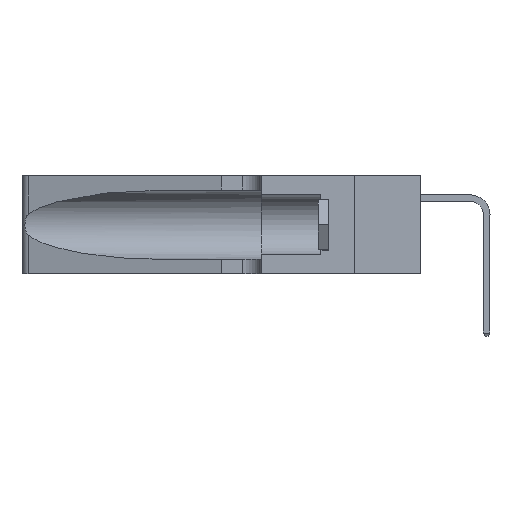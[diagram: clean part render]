
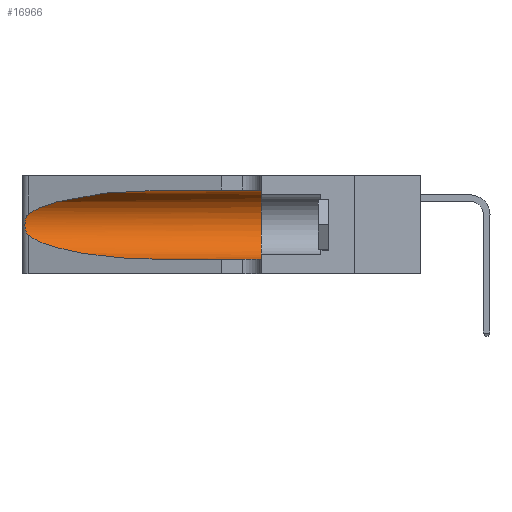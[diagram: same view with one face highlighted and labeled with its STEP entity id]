
A CAD part, left-side view. The second image highlights one B-rep face of the part: STEP entity #16966.
In plain terms, the highlighted cylindrical face has radius 3.308 mm (diameter 6.617 mm), a partial arc.
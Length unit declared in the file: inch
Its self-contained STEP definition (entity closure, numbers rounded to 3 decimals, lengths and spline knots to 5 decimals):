
#611 = FACE_OUTER_BOUND ( 'NONE', #4443, .T. ) ;
#822 = EDGE_CURVE ( 'NONE', #9810, #2990, #13252, .T. ) ;
#973 = CARTESIAN_POINT ( 'NONE',  ( 0.26017, 1.23833, 0.17102 ) ) ;
#1221 = B_SPLINE_CURVE_WITH_KNOTS ( 'NONE', 3,
 ( #13715, #10117, #19068, #8324, #20815, #10199, #22566, #11981, #973, #13793, #2864, #15622, #4724, #17380 ),
 .UNSPECIFIED., .F., .F.,
 ( 4, 2, 2, 2, 2, 2, 4 ),
 ( 0., 0.00027, 0.00053, 0.00107, 0.0016, 0.00187, 0.00214 ),
 .UNSPECIFIED. ) ;
#1453 = CARTESIAN_POINT ( 'NONE',  ( 0.25487, 1.22718, 0.14631 ) ) ;
#1502 = CIRCLE ( 'NONE', #5967, 0.13025 ) ;
#2205 = ORIENTED_EDGE ( 'NONE', *, *, #14631, .T. ) ;
#2864 = CARTESIAN_POINT ( 'NONE',  ( 0.25789, 1.23486, 0.15765 ) ) ;
#2990 = VERTEX_POINT ( 'NONE', #14457 ) ;
#3631 = EDGE_CURVE ( 'NONE', #18304, #9810, #9086, .T. ) ;
#3703 = DIRECTION ( 'NONE',  ( 0., -1., 0. ) ) ;
#4443 = EDGE_LOOP ( 'NONE', ( #17193, #2205, #8664, #22446, #21426, #20558 ) ) ;
#4724 = CARTESIAN_POINT ( 'NONE',  ( 0.25555, 1.22993, 0.14849 ) ) ;
#4751 = CARTESIAN_POINT ( 'NONE',  ( 0.1305, 0.72297, 0.31525 ) ) ;
#4884 = CARTESIAN_POINT ( 'NONE',  ( 0.1305, 0.35, 0.185 ) ) ;
#4976 = CYLINDRICAL_SURFACE ( 'NONE', #18227, 0.13025 ) ;
#5122 = CARTESIAN_POINT ( 'NONE',  ( 0.18966, 0.96281, 0.05475 ) ) ;
#5967 = AXIS2_PLACEMENT_3D ( 'NONE', #4884, #17529, #6722 ) ;
#6227 = DIRECTION ( 'NONE',  ( 0., 0., -1. ) ) ;
#6308 = DIRECTION ( 'NONE',  ( 0., -1., 0. ) ) ;
#6593 = CARTESIAN_POINT ( 'NONE',  ( 0.25487, 1.22718, 0.22369 ) ) ;
#6722 = DIRECTION ( 'NONE',  ( 0., 0., 1. ) ) ;
#7075 = DIRECTION ( 'NONE',  ( 0., -1., 0. ) ) ;
#7609 = VECTOR ( 'NONE', #3703, 39.37008 ) ;
#8324 = CARTESIAN_POINT ( 'NONE',  ( 0.25787, 1.23484, 0.2124 ) ) ;
#8351 = CARTESIAN_POINT ( 'NONE',  ( 0.18966, 0.96281, 0.31525 ) ) ;
#8431 = VECTOR ( 'NONE', #7075, 39.37008 ) ;
#8638 =( BOUNDED_CURVE ( )  B_SPLINE_CURVE ( 3, ( #4751, #8351, #11940, #6593 ),
 .UNSPECIFIED., .F., .F. ) 
 B_SPLINE_CURVE_WITH_KNOTS ( ( 4, 4 ),
 ( 1.5708, 2.84003 ),
 .UNSPECIFIED. ) 
 CURVE ( )  GEOMETRIC_REPRESENTATION_ITEM ( )  RATIONAL_B_SPLINE_CURVE ( ( 1., 0.87, 0.87, 1. ) ) 
 REPRESENTATION_ITEM ( '' )  );
#8664 = ORIENTED_EDGE ( 'NONE', *, *, #3631, .T. ) ;
#9086 =( BOUNDED_CURVE ( )  B_SPLINE_CURVE ( 3, ( #1453, #10650, #5122, #14273 ),
 .UNSPECIFIED., .F., .T. ) 
 B_SPLINE_CURVE_WITH_KNOTS ( ( 4, 4 ),
 ( 3.44316, 4.71239 ),
 .UNSPECIFIED. ) 
 CURVE ( )  GEOMETRIC_REPRESENTATION_ITEM ( )  RATIONAL_B_SPLINE_CURVE ( ( 1., 0.87, 0.87, 1. ) ) 
 REPRESENTATION_ITEM ( '' )  );
#9187 = CARTESIAN_POINT ( 'NONE',  ( 0.1305, 1.61858, 0.05475 ) ) ;
#9243 = CARTESIAN_POINT ( 'NONE',  ( 0.1305, 1.61858, 0.31525 ) ) ;
#9810 = VERTEX_POINT ( 'NONE', #19517 ) ;
#10117 = CARTESIAN_POINT ( 'NONE',  ( 0.25555, 1.22994, 0.2215 ) ) ;
#10199 = CARTESIAN_POINT ( 'NONE',  ( 0.26018, 1.23835, 0.19895 ) ) ;
#10286 = EDGE_CURVE ( 'NONE', #22495, #13396, #8638, .T. ) ;
#10600 = CARTESIAN_POINT ( 'NONE',  ( 0.1305, 0.72297, 0.31525 ) ) ;
#10650 = CARTESIAN_POINT ( 'NONE',  ( 0.2373, 1.15595, 0.08982 ) ) ;
#11940 = CARTESIAN_POINT ( 'NONE',  ( 0.2373, 1.15595, 0.28018 ) ) ;
#11981 = CARTESIAN_POINT ( 'NONE',  ( 0.26075, 1.23896, 0.178 ) ) ;
#12438 = LINE ( 'NONE', #9243, #7609 ) ;
#13252 = LINE ( 'NONE', #9187, #8431 ) ;
#13396 = VERTEX_POINT ( 'NONE', #16566 ) ;
#13715 = CARTESIAN_POINT ( 'NONE',  ( 0.25487, 1.22718, 0.22369 ) ) ;
#13793 = CARTESIAN_POINT ( 'NONE',  ( 0.25856, 1.23593, 0.16098 ) ) ;
#14273 = CARTESIAN_POINT ( 'NONE',  ( 0.1305, 0.72297, 0.05475 ) ) ;
#14457 = CARTESIAN_POINT ( 'NONE',  ( 0.1305, 0.35, 0.05475 ) ) ;
#14631 = EDGE_CURVE ( 'NONE', #13396, #18304, #1221, .T. ) ;
#14663 = EDGE_CURVE ( 'NONE', #15704, #2990, #1502, .T. ) ;
#15622 = CARTESIAN_POINT ( 'NONE',  ( 0.25639, 1.23186, 0.15144 ) ) ;
#15704 = VERTEX_POINT ( 'NONE', #22132 ) ;
#16171 = EDGE_CURVE ( 'NONE', #22495, #15704, #12438, .T. ) ;
#16566 = CARTESIAN_POINT ( 'NONE',  ( 0.25487, 1.22718, 0.22369 ) ) ;
#16966 = ADVANCED_FACE ( 'NONE', ( #611 ), #4976, .F. ) ;
#17193 = ORIENTED_EDGE ( 'NONE', *, *, #10286, .T. ) ;
#17380 = CARTESIAN_POINT ( 'NONE',  ( 0.25487, 1.22718, 0.14631 ) ) ;
#17529 = DIRECTION ( 'NONE',  ( 0., 1., 0. ) ) ;
#18227 = AXIS2_PLACEMENT_3D ( 'NONE', #18884, #6308, #6227 ) ;
#18304 = VERTEX_POINT ( 'NONE', #20230 ) ;
#18884 = CARTESIAN_POINT ( 'NONE',  ( 0.1305, 1.61858, 0.185 ) ) ;
#19068 = CARTESIAN_POINT ( 'NONE',  ( 0.25639, 1.23184, 0.21858 ) ) ;
#19517 = CARTESIAN_POINT ( 'NONE',  ( 0.1305, 0.72297, 0.05475 ) ) ;
#20230 = CARTESIAN_POINT ( 'NONE',  ( 0.25487, 1.22718, 0.14631 ) ) ;
#20558 = ORIENTED_EDGE ( 'NONE', *, *, #16171, .F. ) ;
#20815 = CARTESIAN_POINT ( 'NONE',  ( 0.25854, 1.2359, 0.20912 ) ) ;
#21426 = ORIENTED_EDGE ( 'NONE', *, *, #14663, .F. ) ;
#22132 = CARTESIAN_POINT ( 'NONE',  ( 0.1305, 0.35, 0.31525 ) ) ;
#22446 = ORIENTED_EDGE ( 'NONE', *, *, #822, .T. ) ;
#22495 = VERTEX_POINT ( 'NONE', #10600 ) ;
#22566 = CARTESIAN_POINT ( 'NONE',  ( 0.26075, 1.23896, 0.19203 ) ) ;
